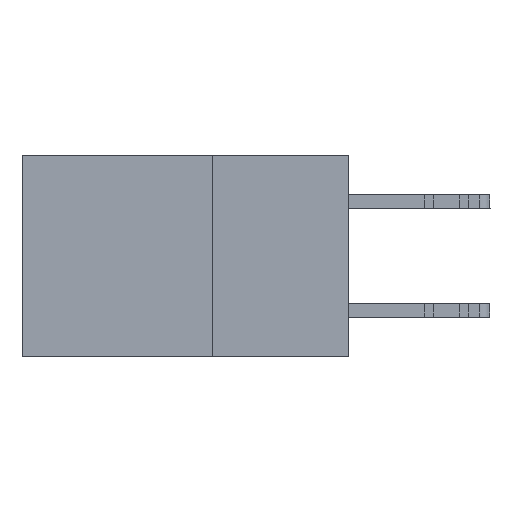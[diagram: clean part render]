
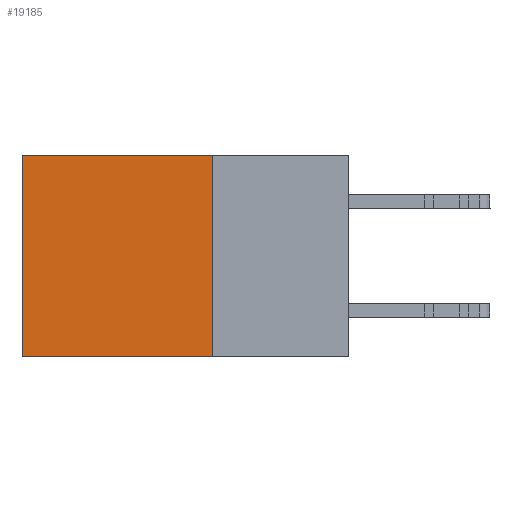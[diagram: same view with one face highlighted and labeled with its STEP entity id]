
A CAD part, left-side view. The second image highlights one B-rep face of the part: STEP entity #19185.
In plain terms, the highlighted planar face has unit normal (-1, 0, 0).
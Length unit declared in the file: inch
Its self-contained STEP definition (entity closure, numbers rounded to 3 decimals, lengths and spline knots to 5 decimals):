
#453 = EDGE_CURVE ( 'NONE', #21775, #11291, #9576, .T. ) ;
#1255 = VECTOR ( 'NONE', #12081, 39.37008 ) ;
#2814 = LINE ( 'NONE', #16288, #14321 ) ;
#4402 = DIRECTION ( 'NONE',  ( 0., 0., -1. ) ) ;
#4725 = DIRECTION ( 'NONE',  ( 0., 0., -1. ) ) ;
#4883 = LINE ( 'NONE', #23024, #28630 ) ;
#5286 = CARTESIAN_POINT ( 'NONE',  ( 0.298, 0.6, -0.37 ) ) ;
#8800 = VERTEX_POINT ( 'NONE', #10541 ) ;
#9576 = LINE ( 'NONE', #10143, #27895 ) ;
#10143 = CARTESIAN_POINT ( 'NONE',  ( 0.298, 0.6, 0. ) ) ;
#10541 = CARTESIAN_POINT ( 'NONE',  ( 0.298, 0.25, -0.37 ) ) ;
#11291 = VERTEX_POINT ( 'NONE', #5286 ) ;
#11888 = CARTESIAN_POINT ( 'NONE',  ( 0.298, 0.25, 0. ) ) ;
#11903 = VERTEX_POINT ( 'NONE', #11888 ) ;
#12081 = DIRECTION ( 'NONE',  ( 0., 1., 0. ) ) ;
#14321 = VECTOR ( 'NONE', #20900, 39.37008 ) ;
#15880 = CARTESIAN_POINT ( 'NONE',  ( 0.298, 0.25, 0. ) ) ;
#16074 = EDGE_LOOP ( 'NONE', ( #25985, #26737, #25111, #17149 ) ) ;
#16288 = CARTESIAN_POINT ( 'NONE',  ( 0.298, 0.25, -0.37 ) ) ;
#17149 = ORIENTED_EDGE ( 'NONE', *, *, #27713, .T. ) ;
#18184 = DIRECTION ( 'NONE',  ( 1., 0., 0. ) ) ;
#18867 = DIRECTION ( 'NONE',  ( 0., 0., -1. ) ) ;
#18906 = LINE ( 'NONE', #21226, #1255 ) ;
#19178 = FACE_OUTER_BOUND ( 'NONE', #16074, .T. ) ;
#19185 = ADVANCED_FACE ( 'NONE', ( #19178 ), #29634, .F. ) ;
#20772 = CARTESIAN_POINT ( 'NONE',  ( 0.298, 0.6, 0. ) ) ;
#20900 = DIRECTION ( 'NONE',  ( 0., 1., 0. ) ) ;
#21226 = CARTESIAN_POINT ( 'NONE',  ( 0.298, 0.25, 0. ) ) ;
#21775 = VERTEX_POINT ( 'NONE', #20772 ) ;
#23024 = CARTESIAN_POINT ( 'NONE',  ( 0.298, 0.25, 0. ) ) ;
#23804 = AXIS2_PLACEMENT_3D ( 'NONE', #15880, #18184, #4402 ) ;
#25111 = ORIENTED_EDGE ( 'NONE', *, *, #27564, .F. ) ;
#25945 = EDGE_CURVE ( 'NONE', #8800, #11291, #2814, .T. ) ;
#25985 = ORIENTED_EDGE ( 'NONE', *, *, #453, .T. ) ;
#26737 = ORIENTED_EDGE ( 'NONE', *, *, #25945, .F. ) ;
#27564 = EDGE_CURVE ( 'NONE', #11903, #8800, #4883, .T. ) ;
#27713 = EDGE_CURVE ( 'NONE', #11903, #21775, #18906, .T. ) ;
#27895 = VECTOR ( 'NONE', #18867, 39.37008 ) ;
#28630 = VECTOR ( 'NONE', #4725, 39.37008 ) ;
#29634 = PLANE ( 'NONE',  #23804 ) ;
